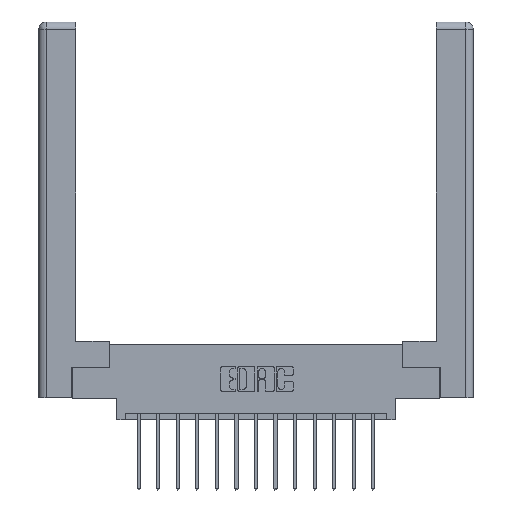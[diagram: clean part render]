
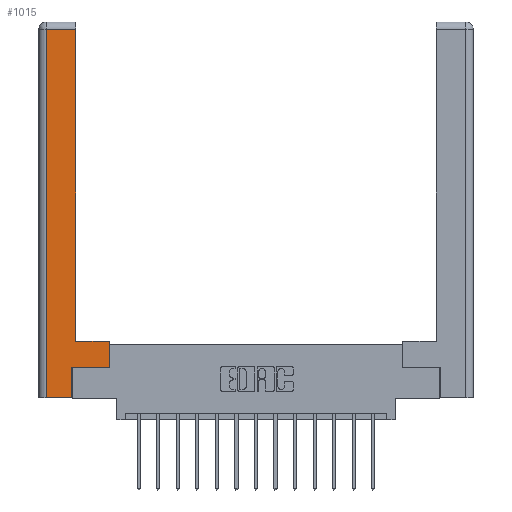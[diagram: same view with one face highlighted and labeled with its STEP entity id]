
A CAD part, top view. The second image highlights one B-rep face of the part: STEP entity #1015.
In plain terms, the highlighted planar face has unit normal (0, 0, 1).
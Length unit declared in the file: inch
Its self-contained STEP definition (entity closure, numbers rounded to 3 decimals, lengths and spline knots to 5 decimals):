
#345 = VECTOR ( 'NONE', #10358, 39.37008 ) ;
#665 = CARTESIAN_POINT ( 'NONE',  ( 0.565, 0.45, 0. ) ) ;
#978 = VERTEX_POINT ( 'NONE', #7154 ) ;
#1015 = ADVANCED_FACE ( 'NONE', ( #8083 ), #4810, .F. ) ;
#1505 = CARTESIAN_POINT ( 'NONE',  ( 0.295, 3., 0. ) ) ;
#1566 = CARTESIAN_POINT ( 'NONE',  ( 0.0615, 0., 0. ) ) ;
#1595 = EDGE_LOOP ( 'NONE', ( #10318, #8941, #15928, #14541, #3249, #3367, #12543, #7257 ) ) ;
#2014 = VECTOR ( 'NONE', #11798, 39.37008 ) ;
#2382 = CARTESIAN_POINT ( 'NONE',  ( 0.565, 0.245, 0. ) ) ;
#3146 = VERTEX_POINT ( 'NONE', #10258 ) ;
#3182 = VERTEX_POINT ( 'NONE', #6571 ) ;
#3249 = ORIENTED_EDGE ( 'NONE', *, *, #3327, .T. ) ;
#3327 = EDGE_CURVE ( 'NONE', #3182, #9533, #15931, .T. ) ;
#3367 = ORIENTED_EDGE ( 'NONE', *, *, #15559, .T. ) ;
#3528 = VECTOR ( 'NONE', #14615, 39.37008 ) ;
#3637 = VERTEX_POINT ( 'NONE', #1566 ) ;
#3642 = DIRECTION ( 'NONE',  ( -1., 0., 0. ) ) ;
#4282 = VERTEX_POINT ( 'NONE', #14166 ) ;
#4630 = VERTEX_POINT ( 'NONE', #2382 ) ;
#4810 = PLANE ( 'NONE',  #13517 ) ;
#4864 = EDGE_CURVE ( 'NONE', #4630, #3146, #9380, .T. ) ;
#5393 = DIRECTION ( 'NONE',  ( 0., 1., 0. ) ) ;
#5912 = EDGE_CURVE ( 'NONE', #3637, #3182, #8940, .T. ) ;
#6165 = VECTOR ( 'NONE', #5393, 39.37008 ) ;
#6571 = CARTESIAN_POINT ( 'NONE',  ( 0.265, 0., 0. ) ) ;
#6896 = VECTOR ( 'NONE', #14719, 39.37008 ) ;
#7154 = CARTESIAN_POINT ( 'NONE',  ( 0.0615, 2.94, 0. ) ) ;
#7257 = ORIENTED_EDGE ( 'NONE', *, *, #13437, .T. ) ;
#7772 = CARTESIAN_POINT ( 'NONE',  ( 0.0615, 2.94, 0. ) ) ;
#8083 = FACE_OUTER_BOUND ( 'NONE', #1595, .T. ) ;
#8369 = LINE ( 'NONE', #1505, #6165 ) ;
#8561 = VERTEX_POINT ( 'NONE', #11049 ) ;
#8940 = LINE ( 'NONE', #11489, #10752 ) ;
#8941 = ORIENTED_EDGE ( 'NONE', *, *, #12872, .T. ) ;
#9380 = LINE ( 'NONE', #665, #3528 ) ;
#9533 = VERTEX_POINT ( 'NONE', #15349 ) ;
#9800 = EDGE_CURVE ( 'NONE', #8561, #4282, #8369, .T. ) ;
#10009 = CARTESIAN_POINT ( 'NONE',  ( 0., 0., 0. ) ) ;
#10258 = CARTESIAN_POINT ( 'NONE',  ( 0.565, 0.45, 0. ) ) ;
#10318 = ORIENTED_EDGE ( 'NONE', *, *, #9800, .T. ) ;
#10358 = DIRECTION ( 'NONE',  ( -1., 0., 0. ) ) ;
#10568 = LINE ( 'NONE', #7772, #345 ) ;
#10722 = CARTESIAN_POINT ( 'NONE',  ( 0.265, 0.245, 0. ) ) ;
#10752 = VECTOR ( 'NONE', #12615, 39.37008 ) ;
#11049 = CARTESIAN_POINT ( 'NONE',  ( 0.295, 0.45, 0. ) ) ;
#11145 = DIRECTION ( 'NONE',  ( -1., 0., 0. ) ) ;
#11234 = VECTOR ( 'NONE', #3642, 39.37008 ) ;
#11304 = VECTOR ( 'NONE', #15546, 39.37008 ) ;
#11489 = CARTESIAN_POINT ( 'NONE',  ( 0.265, 0., 0. ) ) ;
#11798 = DIRECTION ( 'NONE',  ( 0., 1., 0. ) ) ;
#12543 = ORIENTED_EDGE ( 'NONE', *, *, #4864, .T. ) ;
#12615 = DIRECTION ( 'NONE',  ( 1., 0., 0. ) ) ;
#12872 = EDGE_CURVE ( 'NONE', #4282, #978, #10568, .T. ) ;
#13437 = EDGE_CURVE ( 'NONE', #3146, #8561, #13671, .T. ) ;
#13517 = AXIS2_PLACEMENT_3D ( 'NONE', #10009, #13805, #11145 ) ;
#13671 = LINE ( 'NONE', #15255, #11234 ) ;
#13805 = DIRECTION ( 'NONE',  ( 0., 0., -1. ) ) ;
#14166 = CARTESIAN_POINT ( 'NONE',  ( 0.295, 2.94, 0. ) ) ;
#14250 = CARTESIAN_POINT ( 'NONE',  ( 0.565, 0.245, 0. ) ) ;
#14541 = ORIENTED_EDGE ( 'NONE', *, *, #5912, .T. ) ;
#14615 = DIRECTION ( 'NONE',  ( 0., 1., 0. ) ) ;
#14719 = DIRECTION ( 'NONE',  ( 0., -1., 0. ) ) ;
#14753 = LINE ( 'NONE', #14250, #11304 ) ;
#15198 = EDGE_CURVE ( 'NONE', #978, #3637, #16567, .T. ) ;
#15255 = CARTESIAN_POINT ( 'NONE',  ( 0.295, 0.45, 0. ) ) ;
#15349 = CARTESIAN_POINT ( 'NONE',  ( 0.265, 0.245, 0. ) ) ;
#15546 = DIRECTION ( 'NONE',  ( 1., 0., 0. ) ) ;
#15559 = EDGE_CURVE ( 'NONE', #9533, #4630, #14753, .T. ) ;
#15802 = CARTESIAN_POINT ( 'NONE',  ( 0.0615, 0., 0. ) ) ;
#15928 = ORIENTED_EDGE ( 'NONE', *, *, #15198, .T. ) ;
#15931 = LINE ( 'NONE', #10722, #2014 ) ;
#16567 = LINE ( 'NONE', #15802, #6896 ) ;
